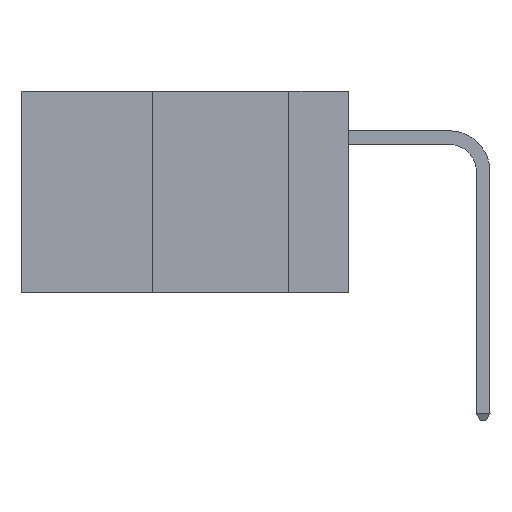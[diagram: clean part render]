
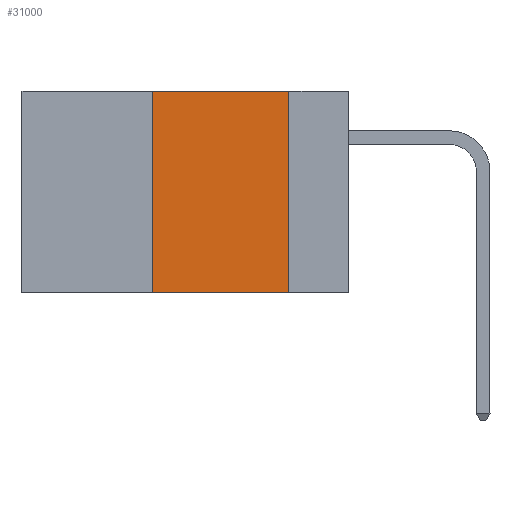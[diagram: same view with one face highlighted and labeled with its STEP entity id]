
A CAD part, left-side view. The second image highlights one B-rep face of the part: STEP entity #31000.
In plain terms, the highlighted planar face has unit normal (-1, 0, 0).
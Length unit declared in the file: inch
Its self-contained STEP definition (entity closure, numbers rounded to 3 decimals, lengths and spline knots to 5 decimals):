
#168 = VERTEX_POINT ( 'NONE', #6328 ) ;
#600 = DIRECTION ( 'NONE',  ( 0., -1., 0. ) ) ;
#911 = CARTESIAN_POINT ( 'NONE',  ( 0., 0.6, -0.37 ) ) ;
#4248 = EDGE_CURVE ( 'NONE', #16100, #31782, #22133, .T. ) ;
#4864 = VERTEX_POINT ( 'NONE', #27647 ) ;
#5542 = EDGE_CURVE ( 'NONE', #4864, #31782, #25217, .T. ) ;
#5791 = PLANE ( 'NONE',  #12275 ) ;
#6328 = CARTESIAN_POINT ( 'NONE',  ( 0., 0.36, 0. ) ) ;
#8102 = ORIENTED_EDGE ( 'NONE', *, *, #9111, .F. ) ;
#8653 = DIRECTION ( 'NONE',  ( 0., 0., 1. ) ) ;
#9111 = EDGE_CURVE ( 'NONE', #4864, #168, #11255, .T. ) ;
#10835 = CARTESIAN_POINT ( 'NONE',  ( 0., 0.6, 0. ) ) ;
#10922 = VECTOR ( 'NONE', #600, 39.37008 ) ;
#11255 = LINE ( 'NONE', #13712, #26761 ) ;
#11848 = DIRECTION ( 'NONE',  ( 0., 0., -1. ) ) ;
#12036 = ORIENTED_EDGE ( 'NONE', *, *, #18146, .F. ) ;
#12275 = AXIS2_PLACEMENT_3D ( 'NONE', #10835, #15744, #30600 ) ;
#13024 = VECTOR ( 'NONE', #11848, 39.37008 ) ;
#13359 = ORIENTED_EDGE ( 'NONE', *, *, #4248, .F. ) ;
#13712 = CARTESIAN_POINT ( 'NONE',  ( 0., 0.36, 0. ) ) ;
#15744 = DIRECTION ( 'NONE',  ( 1., 0., 0. ) ) ;
#16100 = VERTEX_POINT ( 'NONE', #27223 ) ;
#17563 = VECTOR ( 'NONE', #29603, 39.37008 ) ;
#18146 = EDGE_CURVE ( 'NONE', #168, #16100, #29772, .T. ) ;
#19635 = CARTESIAN_POINT ( 'NONE',  ( 0., 0.6, 0. ) ) ;
#19851 = CARTESIAN_POINT ( 'NONE',  ( 0., 0.11, 0. ) ) ;
#20638 = FACE_OUTER_BOUND ( 'NONE', #28491, .T. ) ;
#22133 = LINE ( 'NONE', #19851, #13024 ) ;
#25217 = LINE ( 'NONE', #911, #10922 ) ;
#26436 = ORIENTED_EDGE ( 'NONE', *, *, #5542, .T. ) ;
#26761 = VECTOR ( 'NONE', #8653, 39.37008 ) ;
#27223 = CARTESIAN_POINT ( 'NONE',  ( 0., 0.11, 0. ) ) ;
#27647 = CARTESIAN_POINT ( 'NONE',  ( 0., 0.36, -0.37 ) ) ;
#28491 = EDGE_LOOP ( 'NONE', ( #13359, #12036, #8102, #26436 ) ) ;
#29603 = DIRECTION ( 'NONE',  ( 0., -1., 0. ) ) ;
#29772 = LINE ( 'NONE', #19635, #17563 ) ;
#30313 = CARTESIAN_POINT ( 'NONE',  ( 0., 0.11, -0.37 ) ) ;
#30600 = DIRECTION ( 'NONE',  ( 0., 0., -1. ) ) ;
#31000 = ADVANCED_FACE ( 'NONE', ( #20638 ), #5791, .F. ) ;
#31782 = VERTEX_POINT ( 'NONE', #30313 ) ;
